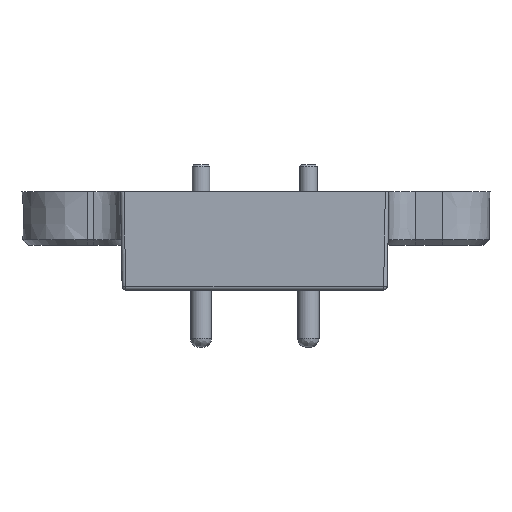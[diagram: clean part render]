
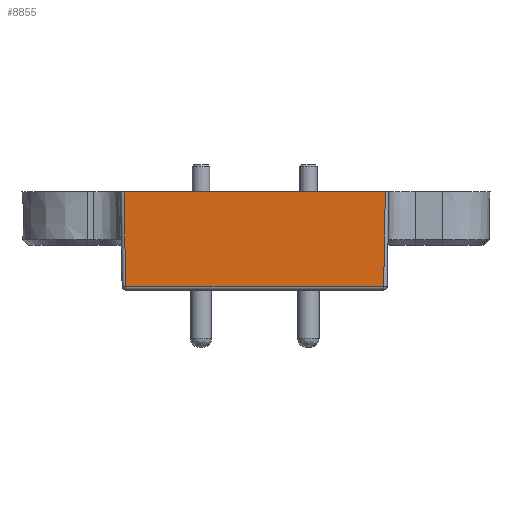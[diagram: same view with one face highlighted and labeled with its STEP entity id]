
A CAD part, left-side view. The second image highlights one B-rep face of the part: STEP entity #8855.
In plain terms, the highlighted planar face has unit normal (-1, 0, -0.018).
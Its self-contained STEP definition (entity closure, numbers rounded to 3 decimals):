
#262 = VERTEX_POINT ( 'NONE', #1621 ) ;
#385 = DIRECTION ( 'NONE',  ( 0., 1., 0. ) ) ;
#878 = CARTESIAN_POINT ( 'NONE',  ( -17., 7.3, 15.9 ) ) ;
#1315 = ORIENTED_EDGE ( 'NONE', *, *, #7398, .T. ) ;
#1621 = CARTESIAN_POINT ( 'NONE',  ( -16.907, 7.207, 10.597 ) ) ;
#1674 = EDGE_CURVE ( 'NONE', #5687, #262, #9586, .T. ) ;
#1766 = VECTOR ( 'NONE', #4735, 1000. ) ;
#1955 = DIRECTION ( 'NONE',  ( 0., -1., 0. ) ) ;
#2859 = EDGE_CURVE ( 'NONE', #262, #5041, #6777, .T. ) ;
#3152 = CARTESIAN_POINT ( 'NONE',  ( -16.907, -7.207, 10.597 ) ) ;
#3665 = ORIENTED_EDGE ( 'NONE', *, *, #2859, .T. ) ;
#3704 = DIRECTION ( 'NONE',  ( 1., 0., 0.017 ) ) ;
#4669 = FACE_OUTER_BOUND ( 'NONE', #7450, .T. ) ;
#4735 = DIRECTION ( 'NONE',  ( 0.017, -0.017, -1. ) ) ;
#4760 = VECTOR ( 'NONE', #385, 1000. ) ;
#5041 = VERTEX_POINT ( 'NONE', #11375 ) ;
#5172 = LINE ( 'NONE', #9074, #4760 ) ;
#5687 = VERTEX_POINT ( 'NONE', #7211 ) ;
#6351 = ORIENTED_EDGE ( 'NONE', *, *, #1674, .T. ) ;
#6436 = EDGE_CURVE ( 'NONE', #7316, #5687, #5172, .T. ) ;
#6777 = LINE ( 'NONE', #10677, #10815 ) ;
#6855 = CARTESIAN_POINT ( 'NONE',  ( -17., -7.3, 15.9 ) ) ;
#7049 = DIRECTION ( 'NONE',  ( -0.017, -0.017, 1. ) ) ;
#7211 = CARTESIAN_POINT ( 'NONE',  ( -17., 7.3, 15.9 ) ) ;
#7316 = VERTEX_POINT ( 'NONE', #6855 ) ;
#7398 = EDGE_CURVE ( 'NONE', #5041, #7316, #11888, .T. ) ;
#7450 = EDGE_LOOP ( 'NONE', ( #9852, #6351, #3665, #1315 ) ) ;
#7611 = DIRECTION ( 'NONE',  ( 0., -1., 0. ) ) ;
#8570 = PLANE ( 'NONE',  #12190 ) ;
#8855 = ADVANCED_FACE ( 'NONE', ( #4669 ), #8570, .F. ) ;
#9074 = CARTESIAN_POINT ( 'NONE',  ( -17., -7.3, 15.9 ) ) ;
#9586 = LINE ( 'NONE', #878, #1766 ) ;
#9852 = ORIENTED_EDGE ( 'NONE', *, *, #6436, .T. ) ;
#10107 = VECTOR ( 'NONE', #7049, 1000. ) ;
#10677 = CARTESIAN_POINT ( 'NONE',  ( -16.907, 7.207, 10.597 ) ) ;
#10815 = VECTOR ( 'NONE', #1955, 1000. ) ;
#11375 = CARTESIAN_POINT ( 'NONE',  ( -16.907, -7.207, 10.597 ) ) ;
#11888 = LINE ( 'NONE', #3152, #10107 ) ;
#12190 = AXIS2_PLACEMENT_3D ( 'NONE', #12447, #3704, #7611 ) ;
#12447 = CARTESIAN_POINT ( 'NONE',  ( -16.954, 0., 13.248 ) ) ;
